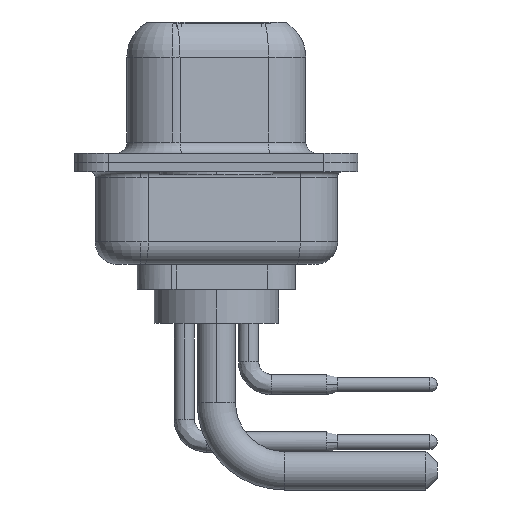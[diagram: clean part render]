
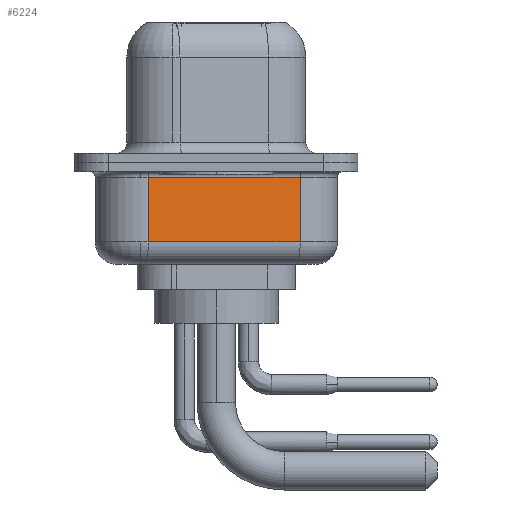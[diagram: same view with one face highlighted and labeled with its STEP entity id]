
A CAD part, left-side view. The second image highlights one B-rep face of the part: STEP entity #6224.
In plain terms, the highlighted planar face has unit normal (-0.985, -0.174, 0).
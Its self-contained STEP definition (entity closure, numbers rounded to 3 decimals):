
#439 = EDGE_LOOP ( 'NONE', ( #15156, #3977, #7890, #1436 ) ) ;
#477 = CARTESIAN_POINT ( 'NONE',  ( 2.855, 3.003, -3.5 ) ) ;
#1024 = DIRECTION ( 'NONE',  ( -0.174, 0.985, 0. ) ) ;
#1436 = ORIENTED_EDGE ( 'NONE', *, *, #12119, .T. ) ;
#2130 = FACE_OUTER_BOUND ( 'NONE', #439, .T. ) ;
#2881 = VERTEX_POINT ( 'NONE', #10320 ) ;
#3648 = VERTEX_POINT ( 'NONE', #8955 ) ;
#3977 = ORIENTED_EDGE ( 'NONE', *, *, #7634, .T. ) ;
#4248 = CARTESIAN_POINT ( 'NONE',  ( 2.855, 3.003, -0.65 ) ) ;
#4420 = VECTOR ( 'NONE', #14782, 1000. ) ;
#4790 = AXIS2_PLACEMENT_3D ( 'NONE', #13098, #15438, #1024 ) ;
#5049 = DIRECTION ( 'NONE',  ( 0.174, -0.985, 0. ) ) ;
#5069 = VECTOR ( 'NONE', #5049, 1000. ) ;
#5164 = VECTOR ( 'NONE', #12290, 1000. ) ;
#5858 = CARTESIAN_POINT ( 'NONE',  ( 2.855, 3.003, -0.65 ) ) ;
#6224 = ADVANCED_FACE ( 'NONE', ( #2130 ), #11846, .F. ) ;
#7446 = LINE ( 'NONE', #14558, #5164 ) ;
#7634 = EDGE_CURVE ( 'NONE', #2881, #3648, #13396, .T. ) ;
#7890 = ORIENTED_EDGE ( 'NONE', *, *, #12055, .T. ) ;
#8446 = VERTEX_POINT ( 'NONE', #5858 ) ;
#8937 = VERTEX_POINT ( 'NONE', #9350 ) ;
#8955 = CARTESIAN_POINT ( 'NONE',  ( 4.037, -3.697, -3.5 ) ) ;
#9350 = CARTESIAN_POINT ( 'NONE',  ( 4.037, -3.697, -0.65 ) ) ;
#10320 = CARTESIAN_POINT ( 'NONE',  ( 2.855, 3.003, -3.5 ) ) ;
#11846 = PLANE ( 'NONE',  #4790 ) ;
#12055 = EDGE_CURVE ( 'NONE', #3648, #8937, #7446, .T. ) ;
#12119 = EDGE_CURVE ( 'NONE', #8937, #8446, #12370, .T. ) ;
#12159 = EDGE_CURVE ( 'NONE', #2881, #8446, #12730, .T. ) ;
#12290 = DIRECTION ( 'NONE',  ( 0., 0., 1. ) ) ;
#12370 = LINE ( 'NONE', #4248, #4420 ) ;
#12494 = CARTESIAN_POINT ( 'NONE',  ( 2.855, 3.003, -4.5 ) ) ;
#12730 = LINE ( 'NONE', #12494, #15148 ) ;
#13098 = CARTESIAN_POINT ( 'NONE',  ( 2.855, 3.003, -4.5 ) ) ;
#13396 = LINE ( 'NONE', #477, #5069 ) ;
#13654 = DIRECTION ( 'NONE',  ( 0., 0., 1. ) ) ;
#14558 = CARTESIAN_POINT ( 'NONE',  ( 4.037, -3.697, -4.5 ) ) ;
#14782 = DIRECTION ( 'NONE',  ( -0.174, 0.985, 0. ) ) ;
#15148 = VECTOR ( 'NONE', #13654, 1000. ) ;
#15156 = ORIENTED_EDGE ( 'NONE', *, *, #12159, .F. ) ;
#15438 = DIRECTION ( 'NONE',  ( 0.985, 0.174, 0. ) ) ;
